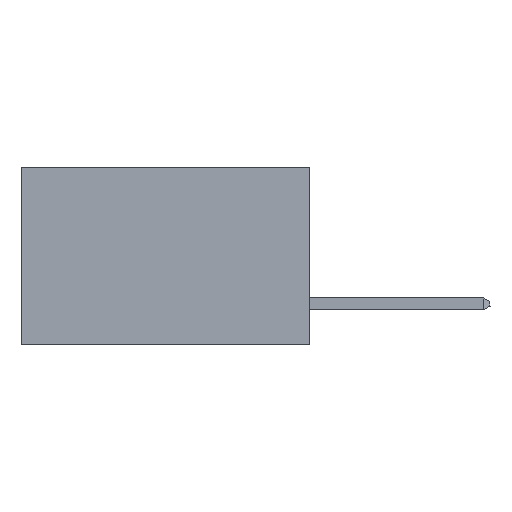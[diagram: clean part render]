
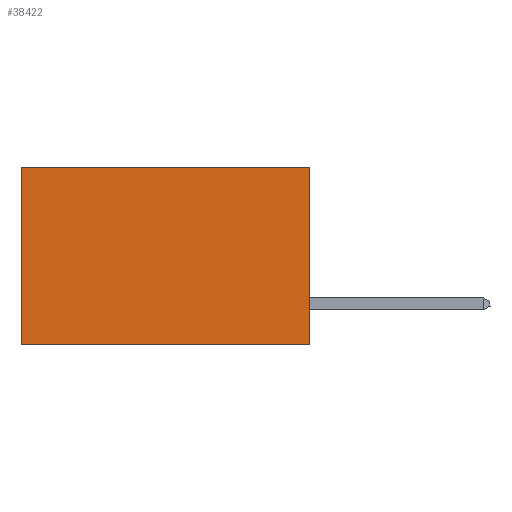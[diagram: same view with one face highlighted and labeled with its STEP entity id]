
A CAD part, left-side view. The second image highlights one B-rep face of the part: STEP entity #38422.
In plain terms, the highlighted planar face has unit normal (-1, 0, 0).
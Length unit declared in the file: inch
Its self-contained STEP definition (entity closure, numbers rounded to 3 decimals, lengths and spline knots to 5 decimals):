
#1089 = EDGE_LOOP ( 'NONE', ( #12072, #26117, #39571, #1170 ) ) ;
#1170 = ORIENTED_EDGE ( 'NONE', *, *, #17313, .T. ) ;
#3094 = VECTOR ( 'NONE', #44895, 39.37008 ) ;
#7789 = FACE_OUTER_BOUND ( 'NONE', #1089, .T. ) ;
#12072 = ORIENTED_EDGE ( 'NONE', *, *, #17754, .T. ) ;
#15134 = VERTEX_POINT ( 'NONE', #41485 ) ;
#15484 = CARTESIAN_POINT ( 'NONE',  ( 0.2875, 0.6, 0. ) ) ;
#16657 = CARTESIAN_POINT ( 'NONE',  ( 0.2875, 0., 0. ) ) ;
#17313 = EDGE_CURVE ( 'NONE', #32153, #46511, #32378, .T. ) ;
#17754 = EDGE_CURVE ( 'NONE', #46511, #15134, #47495, .T. ) ;
#19728 = CARTESIAN_POINT ( 'NONE',  ( 0.2875, 0., 0. ) ) ;
#21016 = LINE ( 'NONE', #37253, #3094 ) ;
#21330 = DIRECTION ( 'NONE',  ( 0., 1., 0. ) ) ;
#21442 = LINE ( 'NONE', #19728, #28220 ) ;
#25960 = EDGE_CURVE ( 'NONE', #26323, #15134, #21016, .T. ) ;
#26117 = ORIENTED_EDGE ( 'NONE', *, *, #25960, .F. ) ;
#26323 = VERTEX_POINT ( 'NONE', #27768 ) ;
#27462 = PLANE ( 'NONE',  #36016 ) ;
#27768 = CARTESIAN_POINT ( 'NONE',  ( 0.2875, 0., -0.37 ) ) ;
#28220 = VECTOR ( 'NONE', #42181, 39.37008 ) ;
#31805 = VECTOR ( 'NONE', #21330, 39.37008 ) ;
#32153 = VERTEX_POINT ( 'NONE', #41116 ) ;
#32378 = LINE ( 'NONE', #16657, #31805 ) ;
#34279 = DIRECTION ( 'NONE',  ( 0., 0., -1. ) ) ;
#34943 = DIRECTION ( 'NONE',  ( 0., 0., -1. ) ) ;
#36016 = AXIS2_PLACEMENT_3D ( 'NONE', #46003, #46158, #34943 ) ;
#36659 = CARTESIAN_POINT ( 'NONE',  ( 0.2875, 0.6, 0. ) ) ;
#37253 = CARTESIAN_POINT ( 'NONE',  ( 0.2875, 0., -0.37 ) ) ;
#37787 = EDGE_CURVE ( 'NONE', #32153, #26323, #21442, .T. ) ;
#38422 = ADVANCED_FACE ( 'NONE', ( #7789 ), #27462, .F. ) ;
#39354 = VECTOR ( 'NONE', #34279, 39.37008 ) ;
#39571 = ORIENTED_EDGE ( 'NONE', *, *, #37787, .F. ) ;
#41116 = CARTESIAN_POINT ( 'NONE',  ( 0.2875, 0., 0. ) ) ;
#41485 = CARTESIAN_POINT ( 'NONE',  ( 0.2875, 0.6, -0.37 ) ) ;
#42181 = DIRECTION ( 'NONE',  ( 0., 0., -1. ) ) ;
#44895 = DIRECTION ( 'NONE',  ( 0., 1., 0. ) ) ;
#46003 = CARTESIAN_POINT ( 'NONE',  ( 0.2875, 0., 0. ) ) ;
#46158 = DIRECTION ( 'NONE',  ( 1., 0., 0. ) ) ;
#46511 = VERTEX_POINT ( 'NONE', #36659 ) ;
#47495 = LINE ( 'NONE', #15484, #39354 ) ;
